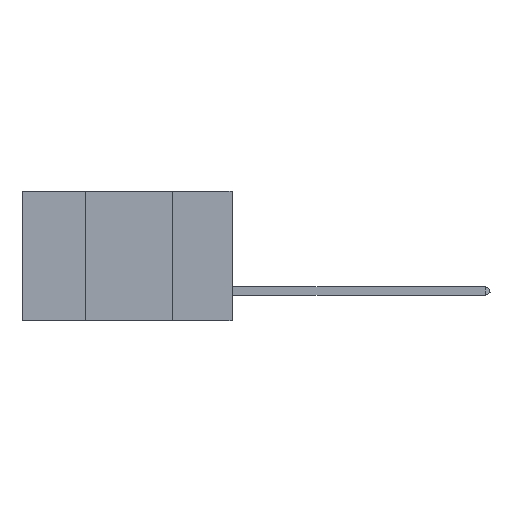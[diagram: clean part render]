
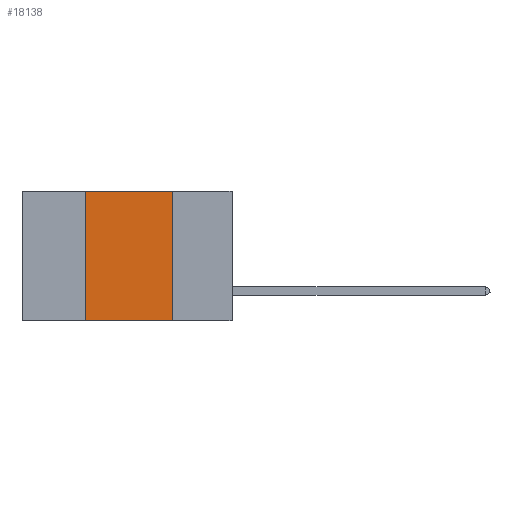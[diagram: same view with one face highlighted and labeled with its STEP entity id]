
A CAD part, left-side view. The second image highlights one B-rep face of the part: STEP entity #18138.
In plain terms, the highlighted planar face has unit normal (-1, 0, 0).
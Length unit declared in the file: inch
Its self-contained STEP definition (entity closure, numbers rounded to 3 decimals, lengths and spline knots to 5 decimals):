
#661 = ORIENTED_EDGE ( 'NONE', *, *, #25191, .T. ) ;
#795 = PLANE ( 'NONE',  #11819 ) ;
#1000 = EDGE_LOOP ( 'NONE', ( #7336, #28077, #13237, #661 ) ) ;
#2188 = VERTEX_POINT ( 'NONE', #15120 ) ;
#3197 = DIRECTION ( 'NONE',  ( 0., 0., -1. ) ) ;
#3731 = CARTESIAN_POINT ( 'NONE',  ( 0., 0.6, 0. ) ) ;
#6382 = DIRECTION ( 'NONE',  ( 0., 0., -1. ) ) ;
#6384 = EDGE_CURVE ( 'NONE', #20710, #27356, #29615, .T. ) ;
#7336 = ORIENTED_EDGE ( 'NONE', *, *, #31890, .F. ) ;
#7666 = VECTOR ( 'NONE', #26858, 39.37008 ) ;
#7690 = CARTESIAN_POINT ( 'NONE',  ( 0., 0.6, -0.37 ) ) ;
#8339 = CARTESIAN_POINT ( 'NONE',  ( 0., 0.42, 0. ) ) ;
#11819 = AXIS2_PLACEMENT_3D ( 'NONE', #16103, #28073, #3197 ) ;
#12100 = VERTEX_POINT ( 'NONE', #32230 ) ;
#13237 = ORIENTED_EDGE ( 'NONE', *, *, #23157, .F. ) ;
#15007 = VECTOR ( 'NONE', #15159, 39.37008 ) ;
#15120 = CARTESIAN_POINT ( 'NONE',  ( 0., 0.42, -0.37 ) ) ;
#15159 = DIRECTION ( 'NONE',  ( 0., -1., 0. ) ) ;
#16092 = DIRECTION ( 'NONE',  ( 0., -1., 0. ) ) ;
#16103 = CARTESIAN_POINT ( 'NONE',  ( 0., 0.6, 0. ) ) ;
#17023 = FACE_OUTER_BOUND ( 'NONE', #1000, .T. ) ;
#18138 = ADVANCED_FACE ( 'NONE', ( #17023 ), #795, .F. ) ;
#20710 = VERTEX_POINT ( 'NONE', #8339 ) ;
#21389 = VECTOR ( 'NONE', #16092, 39.37008 ) ;
#21738 = LINE ( 'NONE', #24568, #7666 ) ;
#22389 = LINE ( 'NONE', #7690, #15007 ) ;
#22698 = CARTESIAN_POINT ( 'NONE',  ( 0., 0.17, 0. ) ) ;
#23157 = EDGE_CURVE ( 'NONE', #2188, #20710, #21738, .T. ) ;
#23346 = VECTOR ( 'NONE', #6382, 39.37008 ) ;
#23483 = CARTESIAN_POINT ( 'NONE',  ( 0., 0.17, 0. ) ) ;
#24568 = CARTESIAN_POINT ( 'NONE',  ( 0., 0.42, 0. ) ) ;
#25191 = EDGE_CURVE ( 'NONE', #2188, #12100, #22389, .T. ) ;
#26858 = DIRECTION ( 'NONE',  ( 0., 0., 1. ) ) ;
#27356 = VERTEX_POINT ( 'NONE', #22698 ) ;
#28073 = DIRECTION ( 'NONE',  ( 1., 0., 0. ) ) ;
#28077 = ORIENTED_EDGE ( 'NONE', *, *, #6384, .F. ) ;
#29601 = LINE ( 'NONE', #23483, #23346 ) ;
#29615 = LINE ( 'NONE', #3731, #21389 ) ;
#31890 = EDGE_CURVE ( 'NONE', #27356, #12100, #29601, .T. ) ;
#32230 = CARTESIAN_POINT ( 'NONE',  ( 0., 0.17, -0.37 ) ) ;
